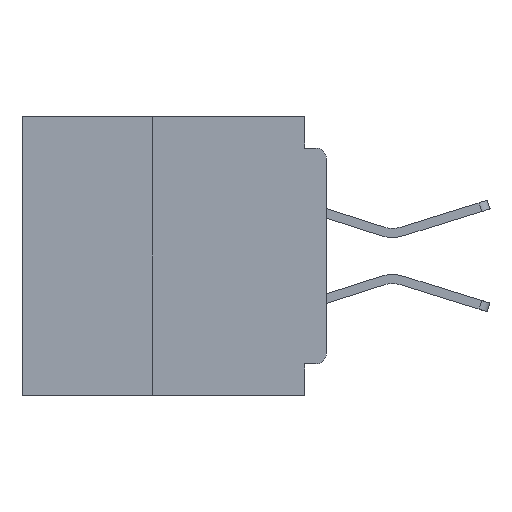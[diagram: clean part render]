
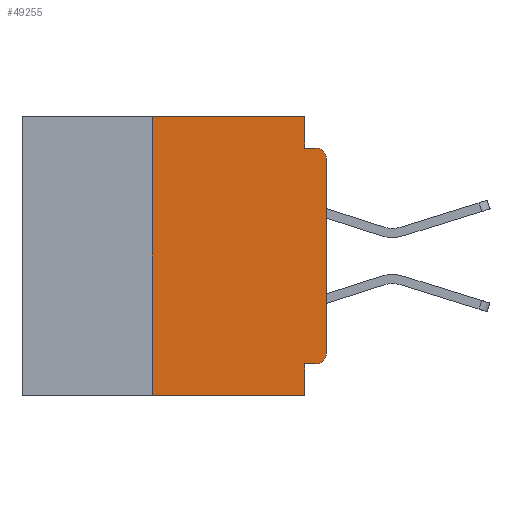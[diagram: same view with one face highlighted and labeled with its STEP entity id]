
A CAD part, left-side view. The second image highlights one B-rep face of the part: STEP entity #49255.
In plain terms, the highlighted planar face has unit normal (-1, 0, 0).
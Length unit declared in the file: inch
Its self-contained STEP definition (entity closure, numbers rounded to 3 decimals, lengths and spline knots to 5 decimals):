
#743 = CIRCLE ( 'NONE', #30090, 0.015 ) ;
#1050 = CIRCLE ( 'NONE', #29652, 0.015 ) ;
#1432 = CARTESIAN_POINT ( 'NONE',  ( 0., 0., -0.355 ) ) ;
#1833 = PLANE ( 'NONE',  #5679 ) ;
#2308 = VECTOR ( 'NONE', #33123, 39.37008 ) ;
#3227 = VERTEX_POINT ( 'NONE', #36791 ) ;
#3324 = VECTOR ( 'NONE', #24811, 39.37008 ) ;
#4510 = CARTESIAN_POINT ( 'NONE',  ( 0., 0.031, 0. ) ) ;
#4777 = ORIENTED_EDGE ( 'NONE', *, *, #33981, .T. ) ;
#5060 = EDGE_CURVE ( 'NONE', #40799, #6744, #24315, .T. ) ;
#5679 = AXIS2_PLACEMENT_3D ( 'NONE', #21301, #13571, #40756 ) ;
#6284 = VECTOR ( 'NONE', #22494, 39.37008 ) ;
#6439 = CARTESIAN_POINT ( 'NONE',  ( 0., 0., -0.06 ) ) ;
#6744 = VERTEX_POINT ( 'NONE', #6439 ) ;
#7753 = CARTESIAN_POINT ( 'NONE',  ( 0., 0.031, -0.4 ) ) ;
#8357 = DIRECTION ( 'NONE',  ( -1., 0., 0. ) ) ;
#8767 = LINE ( 'NONE', #45648, #6284 ) ;
#9806 = VERTEX_POINT ( 'NONE', #4510 ) ;
#10109 = DIRECTION ( 'NONE',  ( -1., 0., 0. ) ) ;
#11174 = VECTOR ( 'NONE', #28585, 39.37008 ) ;
#11911 = CARTESIAN_POINT ( 'NONE',  ( 0., 0.031, -0.355 ) ) ;
#13334 = VERTEX_POINT ( 'NONE', #37507 ) ;
#13571 = DIRECTION ( 'NONE',  ( 1., 0., 0. ) ) ;
#13700 = LINE ( 'NONE', #1432, #3324 ) ;
#14607 = CARTESIAN_POINT ( 'NONE',  ( 0., 0.25, -0.4 ) ) ;
#14810 = VERTEX_POINT ( 'NONE', #11911 ) ;
#15472 = EDGE_CURVE ( 'NONE', #13334, #32734, #44519, .T. ) ;
#18323 = ORIENTED_EDGE ( 'NONE', *, *, #23222, .F. ) ;
#18387 = DIRECTION ( 'NONE',  ( 0., 0., 1. ) ) ;
#18551 = VERTEX_POINT ( 'NONE', #37093 ) ;
#18983 = ORIENTED_EDGE ( 'NONE', *, *, #43455, .F. ) ;
#21301 = CARTESIAN_POINT ( 'NONE',  ( 0., 0.437, 0. ) ) ;
#22311 = CARTESIAN_POINT ( 'NONE',  ( 0., 0.25, 0. ) ) ;
#22494 = DIRECTION ( 'NONE',  ( 0., -1., 0. ) ) ;
#23222 = EDGE_CURVE ( 'NONE', #18551, #40346, #8767, .T. ) ;
#23427 = VECTOR ( 'NONE', #45973, 39.37008 ) ;
#23577 = EDGE_CURVE ( 'NONE', #9806, #18551, #30650, .T. ) ;
#23582 = CARTESIAN_POINT ( 'NONE',  ( 0., 0.031, -0.4 ) ) ;
#24315 = LINE ( 'NONE', #33737, #2308 ) ;
#24811 = DIRECTION ( 'NONE',  ( 0., 1., 0. ) ) ;
#25370 = DIRECTION ( 'NONE',  ( 0., -1., 0. ) ) ;
#25567 = ORIENTED_EDGE ( 'NONE', *, *, #15472, .F. ) ;
#26102 = VERTEX_POINT ( 'NONE', #23582 ) ;
#27249 = VECTOR ( 'NONE', #34956, 39.37008 ) ;
#27628 = ORIENTED_EDGE ( 'NONE', *, *, #37484, .F. ) ;
#28585 = DIRECTION ( 'NONE',  ( 0., 0., -1. ) ) ;
#28960 = ORIENTED_EDGE ( 'NONE', *, *, #45580, .T. ) ;
#29387 = ORIENTED_EDGE ( 'NONE', *, *, #35116, .T. ) ;
#29652 = AXIS2_PLACEMENT_3D ( 'NONE', #31669, #8357, #35535 ) ;
#30090 = AXIS2_PLACEMENT_3D ( 'NONE', #33381, #10109, #37252 ) ;
#30650 = LINE ( 'NONE', #47811, #11174 ) ;
#31669 = CARTESIAN_POINT ( 'NONE',  ( 0., 0.015, -0.06 ) ) ;
#32734 = VERTEX_POINT ( 'NONE', #22311 ) ;
#32835 = EDGE_CURVE ( 'NONE', #32734, #9806, #37914, .T. ) ;
#32948 = CARTESIAN_POINT ( 'NONE',  ( 0., 0.437, -0.4 ) ) ;
#33123 = DIRECTION ( 'NONE',  ( 0., 0., 1. ) ) ;
#33206 = ORIENTED_EDGE ( 'NONE', *, *, #23577, .F. ) ;
#33381 = CARTESIAN_POINT ( 'NONE',  ( 0., 0.015, -0.34 ) ) ;
#33737 = CARTESIAN_POINT ( 'NONE',  ( 0., 0., 0. ) ) ;
#33981 = EDGE_CURVE ( 'NONE', #3227, #40799, #743, .T. ) ;
#34016 = ORIENTED_EDGE ( 'NONE', *, *, #5060, .T. ) ;
#34233 = VECTOR ( 'NONE', #18387, 39.37008 ) ;
#34956 = DIRECTION ( 'NONE',  ( 0., 0., -1. ) ) ;
#35116 = EDGE_CURVE ( 'NONE', #13334, #26102, #50325, .T. ) ;
#35535 = DIRECTION ( 'NONE',  ( 0., 0., -1. ) ) ;
#36791 = CARTESIAN_POINT ( 'NONE',  ( 0., 0.015, -0.355 ) ) ;
#37093 = CARTESIAN_POINT ( 'NONE',  ( 0., 0.031, -0.045 ) ) ;
#37252 = DIRECTION ( 'NONE',  ( 0., 0., -1. ) ) ;
#37484 = EDGE_CURVE ( 'NONE', #14810, #26102, #37488, .T. ) ;
#37488 = LINE ( 'NONE', #7753, #27249 ) ;
#37507 = CARTESIAN_POINT ( 'NONE',  ( 0., 0.25, -0.4 ) ) ;
#37787 = CARTESIAN_POINT ( 'NONE',  ( 0., 0.015, -0.045 ) ) ;
#37914 = LINE ( 'NONE', #41965, #23427 ) ;
#39759 = EDGE_LOOP ( 'NONE', ( #34016, #28960, #18323, #33206, #41098, #25567, #29387, #27628, #18983, #4777 ) ) ;
#40172 = VECTOR ( 'NONE', #25370, 39.37008 ) ;
#40181 = FACE_OUTER_BOUND ( 'NONE', #39759, .T. ) ;
#40346 = VERTEX_POINT ( 'NONE', #37787 ) ;
#40756 = DIRECTION ( 'NONE',  ( 0., 0., -1. ) ) ;
#40799 = VERTEX_POINT ( 'NONE', #44358 ) ;
#41098 = ORIENTED_EDGE ( 'NONE', *, *, #32835, .F. ) ;
#41965 = CARTESIAN_POINT ( 'NONE',  ( 0., 0.437, 0. ) ) ;
#43455 = EDGE_CURVE ( 'NONE', #3227, #14810, #13700, .T. ) ;
#44358 = CARTESIAN_POINT ( 'NONE',  ( 0., 0., -0.34 ) ) ;
#44519 = LINE ( 'NONE', #14607, #34233 ) ;
#45580 = EDGE_CURVE ( 'NONE', #6744, #40346, #1050, .T. ) ;
#45648 = CARTESIAN_POINT ( 'NONE',  ( 0., 0., -0.045 ) ) ;
#45973 = DIRECTION ( 'NONE',  ( 0., -1., 0. ) ) ;
#47811 = CARTESIAN_POINT ( 'NONE',  ( 0., 0.031, 0. ) ) ;
#49255 = ADVANCED_FACE ( 'NONE', ( #40181 ), #1833, .F. ) ;
#50325 = LINE ( 'NONE', #32948, #40172 ) ;
